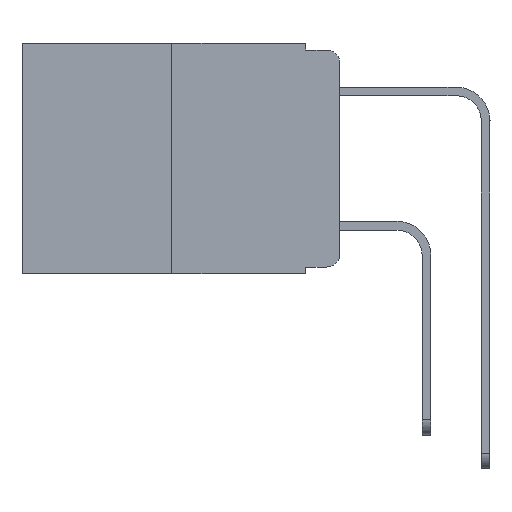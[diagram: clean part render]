
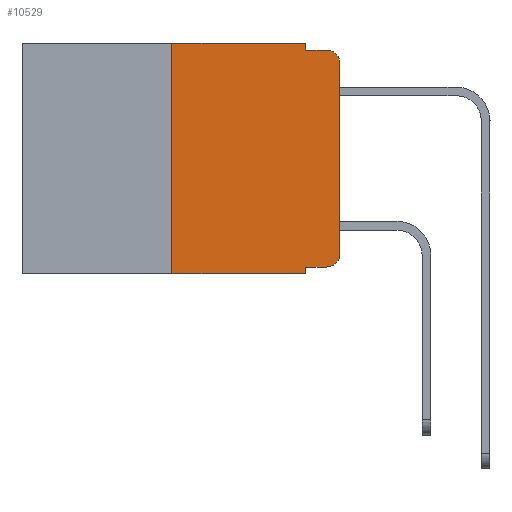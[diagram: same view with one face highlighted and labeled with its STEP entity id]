
A CAD part, left-side view. The second image highlights one B-rep face of the part: STEP entity #10529.
In plain terms, the highlighted planar face has unit normal (-1, 0, 0).
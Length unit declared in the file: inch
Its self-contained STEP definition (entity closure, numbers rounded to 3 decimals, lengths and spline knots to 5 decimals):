
#1403 = ORIENTED_EDGE ( 'NONE', *, *, #18923, .F. ) ;
#1446 = LINE ( 'NONE', #5035, #11216 ) ;
#1498 = ORIENTED_EDGE ( 'NONE', *, *, #18356, .T. ) ;
#1540 = VERTEX_POINT ( 'NONE', #8424 ) ;
#1988 = ORIENTED_EDGE ( 'NONE', *, *, #19465, .T. ) ;
#2363 = AXIS2_PLACEMENT_3D ( 'NONE', #18248, #20093, #8840 ) ;
#2419 = ORIENTED_EDGE ( 'NONE', *, *, #11258, .F. ) ;
#2485 = EDGE_CURVE ( 'NONE', #17015, #3046, #10467, .T. ) ;
#2926 = CARTESIAN_POINT ( 'NONE',  ( 0., 0.051, 0. ) ) ;
#3046 = VERTEX_POINT ( 'NONE', #22049 ) ;
#3242 = ORIENTED_EDGE ( 'NONE', *, *, #20910, .T. ) ;
#3508 = CARTESIAN_POINT ( 'NONE',  ( 0., 0.473, -0.343 ) ) ;
#4069 = VERTEX_POINT ( 'NONE', #23419 ) ;
#4507 = VERTEX_POINT ( 'NONE', #8539 ) ;
#4521 = VERTEX_POINT ( 'NONE', #5875 ) ;
#4754 = DIRECTION ( 'NONE',  ( 0., -1., 0. ) ) ;
#4916 = PLANE ( 'NONE',  #2363 ) ;
#4918 = LINE ( 'NONE', #18529, #14545 ) ;
#5035 = CARTESIAN_POINT ( 'NONE',  ( 0., 0.051, -0.01 ) ) ;
#5238 = FACE_OUTER_BOUND ( 'NONE', #10946, .T. ) ;
#5398 = ORIENTED_EDGE ( 'NONE', *, *, #10492, .F. ) ;
#5834 = VERTEX_POINT ( 'NONE', #10134 ) ;
#5875 = CARTESIAN_POINT ( 'NONE',  ( 0., 0.25, -0.343 ) ) ;
#6112 = ORIENTED_EDGE ( 'NONE', *, *, #2485, .T. ) ;
#7088 = DIRECTION ( 'NONE',  ( 0., -1., 0. ) ) ;
#7187 = DIRECTION ( 'NONE',  ( 0., 0., -1. ) ) ;
#7199 = AXIS2_PLACEMENT_3D ( 'NONE', #19216, #7891, #21040 ) ;
#7311 = AXIS2_PLACEMENT_3D ( 'NONE', #11796, #13842, #15116 ) ;
#7741 = EDGE_CURVE ( 'NONE', #4521, #8334, #21077, .T. ) ;
#7790 = CARTESIAN_POINT ( 'NONE',  ( 0., 0.051, -0.01 ) ) ;
#7891 = DIRECTION ( 'NONE',  ( -1., 0., 0. ) ) ;
#8232 = CARTESIAN_POINT ( 'NONE',  ( 0., 0.25, 0. ) ) ;
#8334 = VERTEX_POINT ( 'NONE', #11138 ) ;
#8424 = CARTESIAN_POINT ( 'NONE',  ( 0., 0., -0.03 ) ) ;
#8539 = CARTESIAN_POINT ( 'NONE',  ( 0., 0.051, 0. ) ) ;
#8840 = DIRECTION ( 'NONE',  ( 0., 0., -1. ) ) ;
#8897 = DIRECTION ( 'NONE',  ( 0., 0., 1. ) ) ;
#9360 = LINE ( 'NONE', #18312, #13827 ) ;
#9375 = DIRECTION ( 'NONE',  ( 0., -1., 0. ) ) ;
#9449 = LINE ( 'NONE', #22946, #13929 ) ;
#9906 = DIRECTION ( 'NONE',  ( 0., 0., 1. ) ) ;
#10059 = VECTOR ( 'NONE', #20467, 39.37008 ) ;
#10134 = CARTESIAN_POINT ( 'NONE',  ( 0., 0.051, -0.333 ) ) ;
#10467 = CIRCLE ( 'NONE', #7311, 0.02 ) ;
#10492 = EDGE_CURVE ( 'NONE', #24056, #4507, #11625, .T. ) ;
#10529 = ADVANCED_FACE ( 'NONE', ( #5238 ), #4916, .F. ) ;
#10946 = EDGE_LOOP ( 'NONE', ( #1988, #3242, #1403, #15894, #5398, #13889, #22868, #2419, #1498, #6112 ) ) ;
#11138 = CARTESIAN_POINT ( 'NONE',  ( 0., 0.051, -0.343 ) ) ;
#11159 = VECTOR ( 'NONE', #16342, 39.37008 ) ;
#11216 = VECTOR ( 'NONE', #7088, 39.37008 ) ;
#11258 = EDGE_CURVE ( 'NONE', #5834, #8334, #4918, .T. ) ;
#11625 = LINE ( 'NONE', #19940, #16039 ) ;
#11796 = CARTESIAN_POINT ( 'NONE',  ( 0., 0.02, -0.313 ) ) ;
#12610 = VERTEX_POINT ( 'NONE', #7790 ) ;
#13009 = CARTESIAN_POINT ( 'NONE',  ( 0., 0.051, -0.333 ) ) ;
#13809 = EDGE_CURVE ( 'NONE', #4507, #12610, #16156, .T. ) ;
#13827 = VECTOR ( 'NONE', #8897, 39.37008 ) ;
#13842 = DIRECTION ( 'NONE',  ( -1., 0., 0. ) ) ;
#13889 = ORIENTED_EDGE ( 'NONE', *, *, #24614, .F. ) ;
#13929 = VECTOR ( 'NONE', #9906, 39.37008 ) ;
#14545 = VECTOR ( 'NONE', #7187, 39.37008 ) ;
#15116 = DIRECTION ( 'NONE',  ( 0., 0., -1. ) ) ;
#15581 = VECTOR ( 'NONE', #9375, 39.37008 ) ;
#15894 = ORIENTED_EDGE ( 'NONE', *, *, #13809, .F. ) ;
#16039 = VECTOR ( 'NONE', #4754, 39.37008 ) ;
#16156 = LINE ( 'NONE', #2926, #11159 ) ;
#16342 = DIRECTION ( 'NONE',  ( 0., 0., -1. ) ) ;
#17015 = VERTEX_POINT ( 'NONE', #21991 ) ;
#18248 = CARTESIAN_POINT ( 'NONE',  ( 0., 0.473, 0. ) ) ;
#18312 = CARTESIAN_POINT ( 'NONE',  ( 0., 0., 0. ) ) ;
#18356 = EDGE_CURVE ( 'NONE', #5834, #17015, #24294, .T. ) ;
#18529 = CARTESIAN_POINT ( 'NONE',  ( 0., 0.051, 0. ) ) ;
#18923 = EDGE_CURVE ( 'NONE', #12610, #4069, #1446, .T. ) ;
#19216 = CARTESIAN_POINT ( 'NONE',  ( 0., 0.02, -0.03 ) ) ;
#19465 = EDGE_CURVE ( 'NONE', #3046, #1540, #9360, .T. ) ;
#19940 = CARTESIAN_POINT ( 'NONE',  ( 0., 0.473, 0. ) ) ;
#20093 = DIRECTION ( 'NONE',  ( 1., 0., 0. ) ) ;
#20467 = DIRECTION ( 'NONE',  ( 0., -1., 0. ) ) ;
#20910 = EDGE_CURVE ( 'NONE', #1540, #4069, #23636, .T. ) ;
#21040 = DIRECTION ( 'NONE',  ( 0., 0., -1. ) ) ;
#21077 = LINE ( 'NONE', #3508, #15581 ) ;
#21991 = CARTESIAN_POINT ( 'NONE',  ( 0., 0.02, -0.333 ) ) ;
#22049 = CARTESIAN_POINT ( 'NONE',  ( 0., 0., -0.313 ) ) ;
#22868 = ORIENTED_EDGE ( 'NONE', *, *, #7741, .T. ) ;
#22946 = CARTESIAN_POINT ( 'NONE',  ( 0., 0.25, 0. ) ) ;
#23419 = CARTESIAN_POINT ( 'NONE',  ( 0., 0.02, -0.01 ) ) ;
#23636 = CIRCLE ( 'NONE', #7199, 0.02 ) ;
#24056 = VERTEX_POINT ( 'NONE', #8232 ) ;
#24294 = LINE ( 'NONE', #13009, #10059 ) ;
#24614 = EDGE_CURVE ( 'NONE', #4521, #24056, #9449, .T. ) ;
